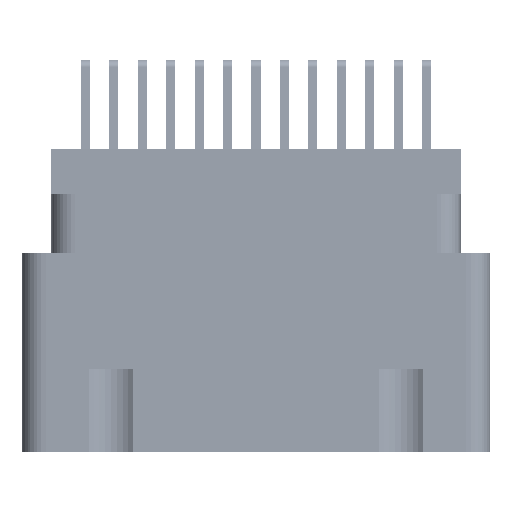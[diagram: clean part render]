
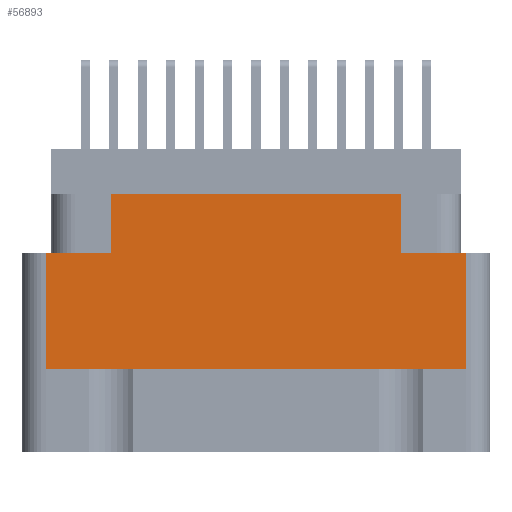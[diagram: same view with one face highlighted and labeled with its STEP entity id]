
A CAD part, left-side view. The second image highlights one B-rep face of the part: STEP entity #56893.
In plain terms, the highlighted planar face has unit normal (-1, 0, 0).
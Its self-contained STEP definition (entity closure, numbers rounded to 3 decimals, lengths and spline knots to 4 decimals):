
#1268 = CARTESIAN_POINT ( 'NONE',  ( -1.359, 0.555, -0.578 ) ) ;
#3391 = CARTESIAN_POINT ( 'NONE',  ( -1.359, 0.617, -0.117 ) ) ;
#3542 = VERTEX_POINT ( 'NONE', #1268 ) ;
#5339 = LINE ( 'NONE', #38991, #53129 ) ;
#6648 = CARTESIAN_POINT ( 'NONE',  ( -1.359, 0.555, -0.798 ) ) ;
#6999 = EDGE_CURVE ( 'NONE', #13841, #15484, #55002, .T. ) ;
#7584 = EDGE_LOOP ( 'NONE', ( #65035, #48754, #55616, #49715, #32686, #51706, #64510, #25286 ) ) ;
#7954 = EDGE_CURVE ( 'NONE', #66529, #53780, #33042, .T. ) ;
#8724 = EDGE_CURVE ( 'NONE', #48189, #53780, #26443, .T. ) ;
#8846 = VECTOR ( 'NONE', #70325, 39.3701 ) ;
#9165 = VERTEX_POINT ( 'NONE', #52813 ) ;
#10130 = DIRECTION ( 'NONE',  ( 0., -1., 0. ) ) ;
#12033 = EDGE_CURVE ( 'NONE', #48189, #34429, #5339, .T. ) ;
#12385 = VECTOR ( 'NONE', #10130, 39.3701 ) ;
#13492 = LINE ( 'NONE', #6648, #36338 ) ;
#13841 = VERTEX_POINT ( 'NONE', #61348 ) ;
#14017 = EDGE_CURVE ( 'NONE', #15484, #34429, #14606, .T. ) ;
#14606 = LINE ( 'NONE', #3391, #8846 ) ;
#15484 = VERTEX_POINT ( 'NONE', #26993 ) ;
#15867 = DIRECTION ( 'NONE',  ( 0., -1., 0. ) ) ;
#17413 = DIRECTION ( 'NONE',  ( 0., 0., 1. ) ) ;
#18649 = CARTESIAN_POINT ( 'NONE',  ( -1.359, -0.3825, -0.117 ) ) ;
#18777 = AXIS2_PLACEMENT_3D ( 'NONE', #59336, #70888, #65116 ) ;
#21057 = CARTESIAN_POINT ( 'NONE',  ( -1.359, -0.555, -0.274 ) ) ;
#23100 = CARTESIAN_POINT ( 'NONE',  ( -1.359, -0.555, -0.578 ) ) ;
#25286 = ORIENTED_EDGE ( 'NONE', *, *, #6999, .F. ) ;
#26443 = LINE ( 'NONE', #59733, #12385 ) ;
#26993 = CARTESIAN_POINT ( 'NONE',  ( -1.359, 0.3825, -0.117 ) ) ;
#27498 = CARTESIAN_POINT ( 'NONE',  ( -1.359, 0.3825, -0.274 ) ) ;
#30036 = VECTOR ( 'NONE', #69858, 39.3701 ) ;
#32227 = LINE ( 'NONE', #60085, #30036 ) ;
#32686 = ORIENTED_EDGE ( 'NONE', *, *, #8724, .F. ) ;
#33042 = LINE ( 'NONE', #39524, #44660 ) ;
#33570 = EDGE_CURVE ( 'NONE', #9165, #3542, #13492, .T. ) ;
#34429 = VERTEX_POINT ( 'NONE', #18649 ) ;
#35859 = FACE_OUTER_BOUND ( 'NONE', #7584, .T. ) ;
#36338 = VECTOR ( 'NONE', #45745, 39.3701 ) ;
#38991 = CARTESIAN_POINT ( 'NONE',  ( -1.359, -0.3825, -0.274 ) ) ;
#39524 = CARTESIAN_POINT ( 'NONE',  ( -1.359, -0.555, -0.798 ) ) ;
#40994 = EDGE_CURVE ( 'NONE', #3542, #66529, #32227, .T. ) ;
#43409 = CARTESIAN_POINT ( 'NONE',  ( -1.359, 0., -0.274 ) ) ;
#44153 = DIRECTION ( 'NONE',  ( 0., 0., 1. ) ) ;
#44660 = VECTOR ( 'NONE', #17413, 39.3701 ) ;
#45745 = DIRECTION ( 'NONE',  ( 0., 0., -1. ) ) ;
#48189 = VERTEX_POINT ( 'NONE', #55261 ) ;
#48754 = ORIENTED_EDGE ( 'NONE', *, *, #33570, .T. ) ;
#48836 = LINE ( 'NONE', #43409, #57680 ) ;
#49715 = ORIENTED_EDGE ( 'NONE', *, *, #7954, .T. ) ;
#50200 = DIRECTION ( 'NONE',  ( 0., 0., 1. ) ) ;
#51187 = EDGE_CURVE ( 'NONE', #9165, #13841, #48836, .T. ) ;
#51350 = VECTOR ( 'NONE', #44153, 39.3701 ) ;
#51706 = ORIENTED_EDGE ( 'NONE', *, *, #12033, .T. ) ;
#52813 = CARTESIAN_POINT ( 'NONE',  ( -1.359, 0.555, -0.274 ) ) ;
#53129 = VECTOR ( 'NONE', #50200, 39.3701 ) ;
#53780 = VERTEX_POINT ( 'NONE', #21057 ) ;
#55002 = LINE ( 'NONE', #27498, #51350 ) ;
#55261 = CARTESIAN_POINT ( 'NONE',  ( -1.359, -0.3825, -0.274 ) ) ;
#55616 = ORIENTED_EDGE ( 'NONE', *, *, #40994, .T. ) ;
#56893 = ADVANCED_FACE ( 'NONE', ( #35859 ), #57920, .T. ) ;
#57680 = VECTOR ( 'NONE', #15867, 39.3701 ) ;
#57920 = PLANE ( 'NONE',  #18777 ) ;
#59336 = CARTESIAN_POINT ( 'NONE',  ( -1.359, -0.617, -0.798 ) ) ;
#59733 = CARTESIAN_POINT ( 'NONE',  ( -1.359, 0., -0.274 ) ) ;
#60085 = CARTESIAN_POINT ( 'NONE',  ( -1.359, 0., -0.578 ) ) ;
#61348 = CARTESIAN_POINT ( 'NONE',  ( -1.359, 0.3825, -0.274 ) ) ;
#64510 = ORIENTED_EDGE ( 'NONE', *, *, #14017, .F. ) ;
#65035 = ORIENTED_EDGE ( 'NONE', *, *, #51187, .F. ) ;
#65116 = DIRECTION ( 'NONE',  ( 0., 0., 1. ) ) ;
#66529 = VERTEX_POINT ( 'NONE', #23100 ) ;
#69858 = DIRECTION ( 'NONE',  ( 0., -1., 0. ) ) ;
#70325 = DIRECTION ( 'NONE',  ( 0., -1., 0. ) ) ;
#70888 = DIRECTION ( 'NONE',  ( -1., 0., 0. ) ) ;
